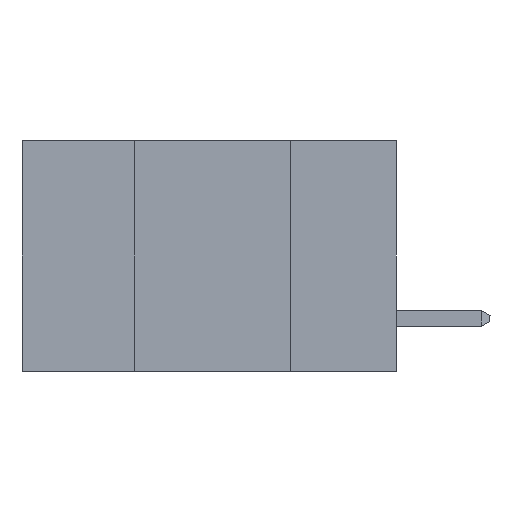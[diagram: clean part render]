
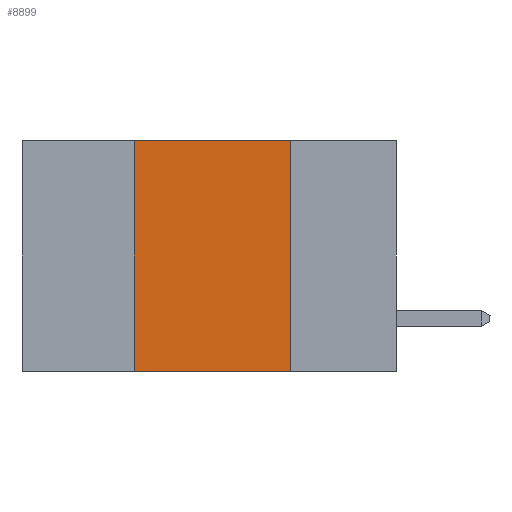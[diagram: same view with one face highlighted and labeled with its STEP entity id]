
A CAD part, left-side view. The second image highlights one B-rep face of the part: STEP entity #8899.
In plain terms, the highlighted planar face has unit normal (-1, 0, 0).
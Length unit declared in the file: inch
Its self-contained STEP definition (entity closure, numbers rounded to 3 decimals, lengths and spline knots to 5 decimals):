
#25 = LINE ( 'NONE', #11078, #4559 ) ;
#140 = EDGE_CURVE ( 'NONE', #2725, #4215, #10540, .T. ) ;
#1041 = VERTEX_POINT ( 'NONE', #10585 ) ;
#1577 = DIRECTION ( 'NONE',  ( 1., 0., 0. ) ) ;
#1618 = DIRECTION ( 'NONE',  ( 0., 0., 1. ) ) ;
#1797 = EDGE_CURVE ( 'NONE', #4215, #5815, #6886, .T. ) ;
#2328 = CARTESIAN_POINT ( 'NONE',  ( 0., 0.6, 0. ) ) ;
#2483 = FACE_OUTER_BOUND ( 'NONE', #10561, .T. ) ;
#2663 = CARTESIAN_POINT ( 'NONE',  ( 0., 0.17, 0. ) ) ;
#2725 = VERTEX_POINT ( 'NONE', #6147 ) ;
#3434 = DIRECTION ( 'NONE',  ( 0., 0., -1. ) ) ;
#3963 = CARTESIAN_POINT ( 'NONE',  ( 0., 0.17, -0.37 ) ) ;
#4155 = LINE ( 'NONE', #5055, #11236 ) ;
#4215 = VERTEX_POINT ( 'NONE', #2663 ) ;
#4279 = ORIENTED_EDGE ( 'NONE', *, *, #140, .F. ) ;
#4428 = DIRECTION ( 'NONE',  ( 0., -1., 0. ) ) ;
#4559 = VECTOR ( 'NONE', #1618, 39.37008 ) ;
#4912 = ORIENTED_EDGE ( 'NONE', *, *, #1797, .F. ) ;
#5055 = CARTESIAN_POINT ( 'NONE',  ( 0., 0.6, -0.37 ) ) ;
#5239 = CARTESIAN_POINT ( 'NONE',  ( 0., 0.6, 0. ) ) ;
#5661 = VECTOR ( 'NONE', #4428, 39.37008 ) ;
#5799 = PLANE ( 'NONE',  #7625 ) ;
#5815 = VERTEX_POINT ( 'NONE', #6690 ) ;
#6147 = CARTESIAN_POINT ( 'NONE',  ( 0., 0.42, 0. ) ) ;
#6299 = ORIENTED_EDGE ( 'NONE', *, *, #6862, .F. ) ;
#6690 = CARTESIAN_POINT ( 'NONE',  ( 0., 0.17, -0.37 ) ) ;
#6834 = ORIENTED_EDGE ( 'NONE', *, *, #7595, .T. ) ;
#6862 = EDGE_CURVE ( 'NONE', #1041, #2725, #25, .T. ) ;
#6886 = LINE ( 'NONE', #3963, #11538 ) ;
#7595 = EDGE_CURVE ( 'NONE', #1041, #5815, #4155, .T. ) ;
#7625 = AXIS2_PLACEMENT_3D ( 'NONE', #5239, #1577, #3434 ) ;
#8899 = ADVANCED_FACE ( 'NONE', ( #2483 ), #5799, .F. ) ;
#10377 = DIRECTION ( 'NONE',  ( 0., 0., -1. ) ) ;
#10540 = LINE ( 'NONE', #2328, #5661 ) ;
#10561 = EDGE_LOOP ( 'NONE', ( #4912, #4279, #6299, #6834 ) ) ;
#10585 = CARTESIAN_POINT ( 'NONE',  ( 0., 0.42, -0.37 ) ) ;
#11078 = CARTESIAN_POINT ( 'NONE',  ( 0., 0.42, -0.37 ) ) ;
#11236 = VECTOR ( 'NONE', #11581, 39.37008 ) ;
#11538 = VECTOR ( 'NONE', #10377, 39.37008 ) ;
#11581 = DIRECTION ( 'NONE',  ( 0., -1., 0. ) ) ;
